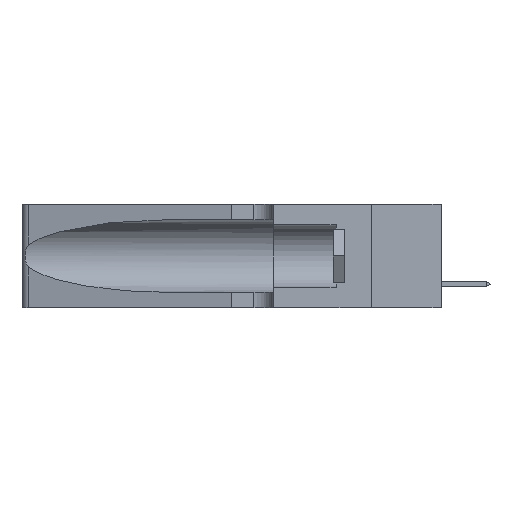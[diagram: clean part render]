
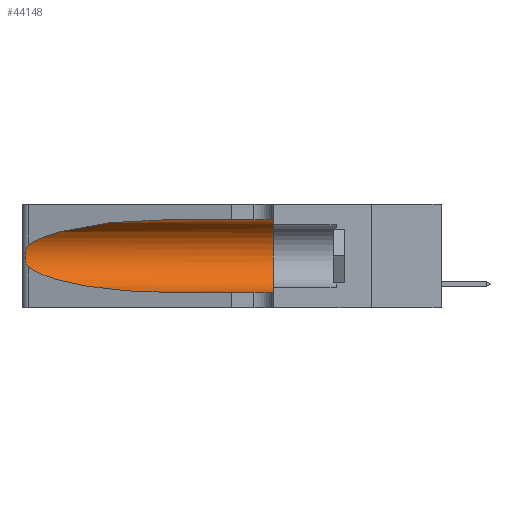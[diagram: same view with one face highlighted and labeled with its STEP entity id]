
A CAD part, left-side view. The second image highlights one B-rep face of the part: STEP entity #44148.
In plain terms, the highlighted cylindrical face has radius 3.308 mm (diameter 6.617 mm), a partial arc.
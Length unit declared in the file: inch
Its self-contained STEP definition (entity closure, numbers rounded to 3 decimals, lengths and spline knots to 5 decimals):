
#594 = CARTESIAN_POINT ( 'NONE',  ( 0.1305, 0.35, 0.31525 ) ) ;
#1166 = EDGE_CURVE ( 'NONE', #41380, #36651, #30337, .T. ) ;
#1491 = B_SPLINE_CURVE_WITH_KNOTS ( 'NONE', 3,
 ( #37687, #33852, #46105, #25614, #9968, #46285, #49942, #18119, #25964, #14298, #29640, #42234, #22111, #2280 ),
 .UNSPECIFIED., .F., .F.,
 ( 4, 2, 2, 2, 2, 2, 4 ),
 ( 0., 0.00027, 0.00053, 0.00107, 0.0016, 0.00187, 0.00214 ),
 .UNSPECIFIED. ) ;
#2108 = ORIENTED_EDGE ( 'NONE', *, *, #48254, .F. ) ;
#2280 = CARTESIAN_POINT ( 'NONE',  ( 0.25487, 1.22718, 0.14631 ) ) ;
#2304 = ORIENTED_EDGE ( 'NONE', *, *, #47478, .T. ) ;
#4245 = VERTEX_POINT ( 'NONE', #594 ) ;
#4278 = AXIS2_PLACEMENT_3D ( 'NONE', #22110, #34213, #29639 ) ;
#8142 = CARTESIAN_POINT ( 'NONE',  ( 0.1305, 0.72297, 0.31525 ) ) ;
#8147 = LINE ( 'NONE', #43986, #49344 ) ;
#8513 = FACE_OUTER_BOUND ( 'NONE', #38817, .T. ) ;
#9234 = DIRECTION ( 'NONE',  ( 0., 0., 1. ) ) ;
#9287 = EDGE_CURVE ( 'NONE', #46799, #41380, #1491, .T. ) ;
#9515 = EDGE_CURVE ( 'NONE', #45128, #46799, #15612, .T. ) ;
#9968 = CARTESIAN_POINT ( 'NONE',  ( 0.25854, 1.2359, 0.20912 ) ) ;
#10686 = ORIENTED_EDGE ( 'NONE', *, *, #9515, .T. ) ;
#11356 = CARTESIAN_POINT ( 'NONE',  ( 0.18966, 0.96281, 0.31525 ) ) ;
#12414 = CARTESIAN_POINT ( 'NONE',  ( 0.1305, 1.61858, 0.05475 ) ) ;
#13143 = VECTOR ( 'NONE', #40363, 39.37008 ) ;
#14298 = CARTESIAN_POINT ( 'NONE',  ( 0.25856, 1.23593, 0.16098 ) ) ;
#14946 = CARTESIAN_POINT ( 'NONE',  ( 0.25487, 1.22718, 0.14631 ) ) ;
#15612 =( BOUNDED_CURVE ( )  B_SPLINE_CURVE ( 3, ( #51523, #11356, #27544, #27867 ),
 .UNSPECIFIED., .F., .F. ) 
 B_SPLINE_CURVE_WITH_KNOTS ( ( 4, 4 ),
 ( 1.5708, 2.84003 ),
 .UNSPECIFIED. ) 
 CURVE ( )  GEOMETRIC_REPRESENTATION_ITEM ( )  RATIONAL_B_SPLINE_CURVE ( ( 1., 0.87, 0.87, 1. ) ) 
 REPRESENTATION_ITEM ( '' )  );
#15700 = CIRCLE ( 'NONE', #38051, 0.13025 ) ;
#15946 = CARTESIAN_POINT ( 'NONE',  ( 0.25487, 1.22718, 0.14631 ) ) ;
#18119 = CARTESIAN_POINT ( 'NONE',  ( 0.26075, 1.23896, 0.178 ) ) ;
#18494 = CARTESIAN_POINT ( 'NONE',  ( 0.1305, 0.72297, 0.05475 ) ) ;
#18659 = CARTESIAN_POINT ( 'NONE',  ( 0.1305, 0.35, 0.05475 ) ) ;
#22110 = CARTESIAN_POINT ( 'NONE',  ( 0.1305, 1.61858, 0.185 ) ) ;
#22111 = CARTESIAN_POINT ( 'NONE',  ( 0.25555, 1.22993, 0.14849 ) ) ;
#23221 = ORIENTED_EDGE ( 'NONE', *, *, #1166, .T. ) ;
#24475 = CARTESIAN_POINT ( 'NONE',  ( 0.18966, 0.96281, 0.05475 ) ) ;
#25614 = CARTESIAN_POINT ( 'NONE',  ( 0.25787, 1.23484, 0.2124 ) ) ;
#25964 = CARTESIAN_POINT ( 'NONE',  ( 0.26017, 1.23833, 0.17102 ) ) ;
#26279 = LINE ( 'NONE', #12414, #13143 ) ;
#27544 = CARTESIAN_POINT ( 'NONE',  ( 0.2373, 1.15595, 0.28018 ) ) ;
#27867 = CARTESIAN_POINT ( 'NONE',  ( 0.25487, 1.22718, 0.22369 ) ) ;
#28942 = CARTESIAN_POINT ( 'NONE',  ( 0.1305, 0.35, 0.185 ) ) ;
#29639 = DIRECTION ( 'NONE',  ( 0., 0., -1. ) ) ;
#29640 = CARTESIAN_POINT ( 'NONE',  ( 0.25789, 1.23486, 0.15765 ) ) ;
#30337 =( BOUNDED_CURVE ( )  B_SPLINE_CURVE ( 3, ( #15946, #32037, #24475, #44573 ),
 .UNSPECIFIED., .F., .F. ) 
 B_SPLINE_CURVE_WITH_KNOTS ( ( 4, 4 ),
 ( 3.44316, 4.71239 ),
 .UNSPECIFIED. ) 
 CURVE ( )  GEOMETRIC_REPRESENTATION_ITEM ( )  RATIONAL_B_SPLINE_CURVE ( ( 1., 0.87, 0.87, 1. ) ) 
 REPRESENTATION_ITEM ( '' )  );
#32037 = CARTESIAN_POINT ( 'NONE',  ( 0.2373, 1.15595, 0.08982 ) ) ;
#33852 = CARTESIAN_POINT ( 'NONE',  ( 0.25555, 1.22994, 0.2215 ) ) ;
#34213 = DIRECTION ( 'NONE',  ( 0., -1., 0. ) ) ;
#34278 = EDGE_CURVE ( 'NONE', #4245, #44313, #15700, .T. ) ;
#36309 = DIRECTION ( 'NONE',  ( 0., 1., 0. ) ) ;
#36651 = VERTEX_POINT ( 'NONE', #18494 ) ;
#37687 = CARTESIAN_POINT ( 'NONE',  ( 0.25487, 1.22718, 0.22369 ) ) ;
#38051 = AXIS2_PLACEMENT_3D ( 'NONE', #28942, #36309, #9234 ) ;
#38260 = ORIENTED_EDGE ( 'NONE', *, *, #9287, .T. ) ;
#38817 = EDGE_LOOP ( 'NONE', ( #10686, #38260, #23221, #2304, #38892, #2108 ) ) ;
#38892 = ORIENTED_EDGE ( 'NONE', *, *, #34278, .F. ) ;
#40363 = DIRECTION ( 'NONE',  ( 0., -1., 0. ) ) ;
#41380 = VERTEX_POINT ( 'NONE', #14946 ) ;
#42234 = CARTESIAN_POINT ( 'NONE',  ( 0.25639, 1.23186, 0.15144 ) ) ;
#43986 = CARTESIAN_POINT ( 'NONE',  ( 0.1305, 1.61858, 0.31525 ) ) ;
#44148 = ADVANCED_FACE ( 'NONE', ( #8513 ), #45288, .F. ) ;
#44313 = VERTEX_POINT ( 'NONE', #18659 ) ;
#44573 = CARTESIAN_POINT ( 'NONE',  ( 0.1305, 0.72297, 0.05475 ) ) ;
#45128 = VERTEX_POINT ( 'NONE', #8142 ) ;
#45288 = CYLINDRICAL_SURFACE ( 'NONE', #4278, 0.13025 ) ;
#46105 = CARTESIAN_POINT ( 'NONE',  ( 0.25639, 1.23184, 0.21858 ) ) ;
#46285 = CARTESIAN_POINT ( 'NONE',  ( 0.26018, 1.23835, 0.19895 ) ) ;
#46799 = VERTEX_POINT ( 'NONE', #50807 ) ;
#47478 = EDGE_CURVE ( 'NONE', #36651, #44313, #26279, .T. ) ;
#48254 = EDGE_CURVE ( 'NONE', #45128, #4245, #8147, .T. ) ;
#48504 = DIRECTION ( 'NONE',  ( 0., -1., 0. ) ) ;
#49344 = VECTOR ( 'NONE', #48504, 39.37008 ) ;
#49942 = CARTESIAN_POINT ( 'NONE',  ( 0.26075, 1.23896, 0.19203 ) ) ;
#50807 = CARTESIAN_POINT ( 'NONE',  ( 0.25487, 1.22718, 0.22369 ) ) ;
#51523 = CARTESIAN_POINT ( 'NONE',  ( 0.1305, 0.72297, 0.31525 ) ) ;
